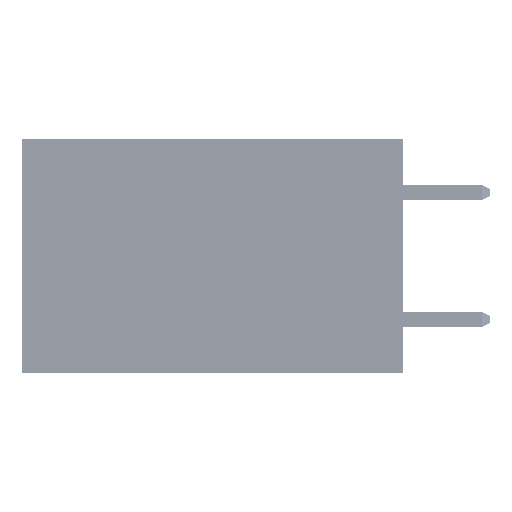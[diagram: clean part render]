
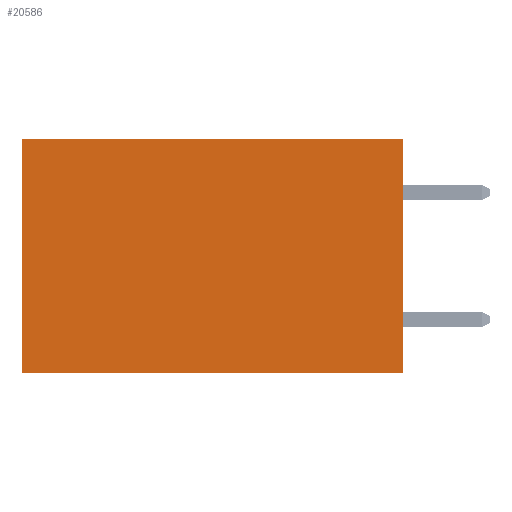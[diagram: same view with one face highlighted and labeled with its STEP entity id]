
A CAD part, left-side view. The second image highlights one B-rep face of the part: STEP entity #20586.
In plain terms, the highlighted planar face has unit normal (-1, 0, 0).
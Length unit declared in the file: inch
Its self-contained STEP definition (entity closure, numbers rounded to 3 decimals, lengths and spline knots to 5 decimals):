
#2742 = ORIENTED_EDGE ( 'NONE', *, *, #6334, .T. ) ;
#3159 = LINE ( 'NONE', #7718, #25013 ) ;
#3655 = ORIENTED_EDGE ( 'NONE', *, *, #39356, .F. ) ;
#5071 = PLANE ( 'NONE',  #31846 ) ;
#6211 = VECTOR ( 'NONE', #48996, 39.37008 ) ;
#6334 = EDGE_CURVE ( 'NONE', #36882, #40442, #3159, .T. ) ;
#6521 = ORIENTED_EDGE ( 'NONE', *, *, #23094, .T. ) ;
#7718 = CARTESIAN_POINT ( 'NONE',  ( 0.2875, 0.6, 0. ) ) ;
#8643 = DIRECTION ( 'NONE',  ( 0., 0., -1. ) ) ;
#10750 = CARTESIAN_POINT ( 'NONE',  ( 0.2875, 0., 0. ) ) ;
#12249 = VECTOR ( 'NONE', #21288, 39.37008 ) ;
#13163 = CARTESIAN_POINT ( 'NONE',  ( 0.2875, 0., 0. ) ) ;
#14202 = CARTESIAN_POINT ( 'NONE',  ( 0.2875, 0., -0.37 ) ) ;
#19305 = LINE ( 'NONE', #10750, #27849 ) ;
#19846 = CARTESIAN_POINT ( 'NONE',  ( 0.2875, 0.6, -0.37 ) ) ;
#20413 = CARTESIAN_POINT ( 'NONE',  ( 0.2875, 0., 0. ) ) ;
#20586 = ADVANCED_FACE ( 'NONE', ( #27759 ), #5071, .F. ) ;
#21093 = ORIENTED_EDGE ( 'NONE', *, *, #34747, .F. ) ;
#21288 = DIRECTION ( 'NONE',  ( 0., 1., 0. ) ) ;
#23094 = EDGE_CURVE ( 'NONE', #44851, #36882, #42092, .T. ) ;
#23729 = CARTESIAN_POINT ( 'NONE',  ( 0.2875, 0.6, 0. ) ) ;
#25013 = VECTOR ( 'NONE', #38824, 39.37008 ) ;
#27759 = FACE_OUTER_BOUND ( 'NONE', #49686, .T. ) ;
#27849 = VECTOR ( 'NONE', #33856, 39.37008 ) ;
#28508 = CARTESIAN_POINT ( 'NONE',  ( 0.2875, 0., 0. ) ) ;
#31846 = AXIS2_PLACEMENT_3D ( 'NONE', #28508, #43999, #8643 ) ;
#32899 = LINE ( 'NONE', #44608, #12249 ) ;
#33856 = DIRECTION ( 'NONE',  ( 0., 0., -1. ) ) ;
#34747 = EDGE_CURVE ( 'NONE', #44851, #43364, #19305, .T. ) ;
#36882 = VERTEX_POINT ( 'NONE', #23729 ) ;
#38824 = DIRECTION ( 'NONE',  ( 0., 0., -1. ) ) ;
#39356 = EDGE_CURVE ( 'NONE', #43364, #40442, #32899, .T. ) ;
#40442 = VERTEX_POINT ( 'NONE', #19846 ) ;
#42092 = LINE ( 'NONE', #13163, #6211 ) ;
#43364 = VERTEX_POINT ( 'NONE', #14202 ) ;
#43999 = DIRECTION ( 'NONE',  ( 1., 0., 0. ) ) ;
#44608 = CARTESIAN_POINT ( 'NONE',  ( 0.2875, 0., -0.37 ) ) ;
#44851 = VERTEX_POINT ( 'NONE', #20413 ) ;
#48996 = DIRECTION ( 'NONE',  ( 0., 1., 0. ) ) ;
#49686 = EDGE_LOOP ( 'NONE', ( #2742, #3655, #21093, #6521 ) ) ;
